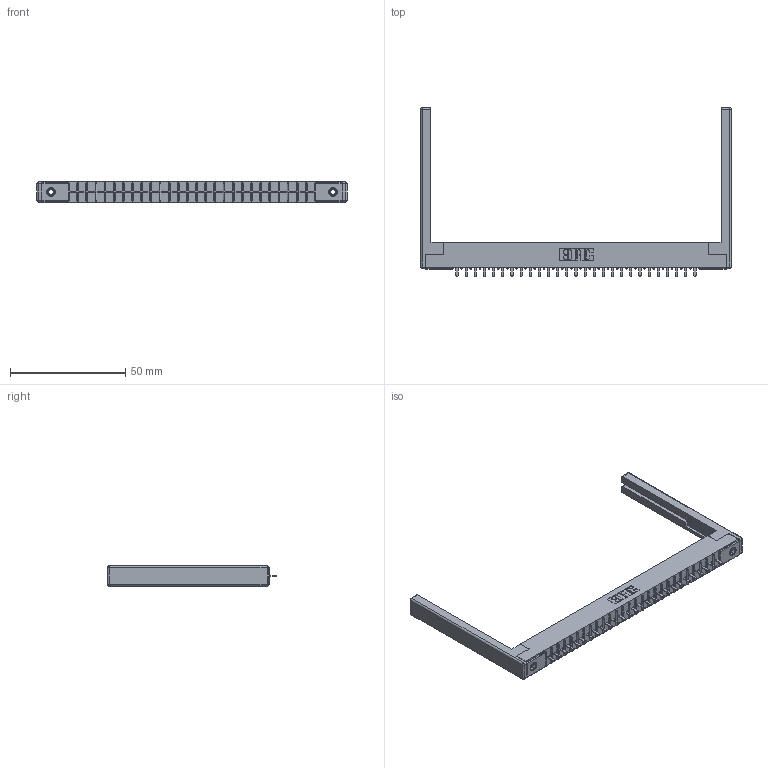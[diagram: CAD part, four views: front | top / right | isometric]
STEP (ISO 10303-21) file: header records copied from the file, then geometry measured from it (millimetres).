
FILE_DESCRIPTION (( 'STEP AP203' ), '1' );
FILE_NAME ('316-027-421-168.STEP', '2020-09-22T23:12:18', ( '' ), ( '' ), 'SwSTEP 2.0', 'SolidWorks 2020', '' );
FILE_SCHEMA (( 'CONFIG_CONTROL_DESIGN' ));
Length unit declared in the file: inch
Products named in the file (5): 307-220-068; 316-027-421-168; 306-290-001_121; 306 Part_.156 Dia; 345-250-001_345-250-001-102
Assembly tree (32 placements, depth 2):
  316-027-421-168
    306 Part_.156 Dia
    306-290-001_121  x27
    345-250-001_345-250-001-102  x2
    307-220-068  x2
Bounding box: 134.42 x 73.18 x 8.71 mm (x, y, z)
Volume: 13732.7 mm3; surface area: 17652.3 mm2
Topology: 32 solids, 32 shells, 2160 faces, 6025 edges, 3850 vertices
Faces by surface type: plane 1425, cylinder 603, sphere 116, cone 12, torus 4
Entity records: 29837 total; most frequent: CARTESIAN_POINT 4973, ORIENTED_EDGE 4920, DIRECTION 4918, EDGE_CURVE 2460, LINE 1912, VECTOR 1912, VERTEX_POINT 1558, AXIS2_PLACEMENT_3D 1503
